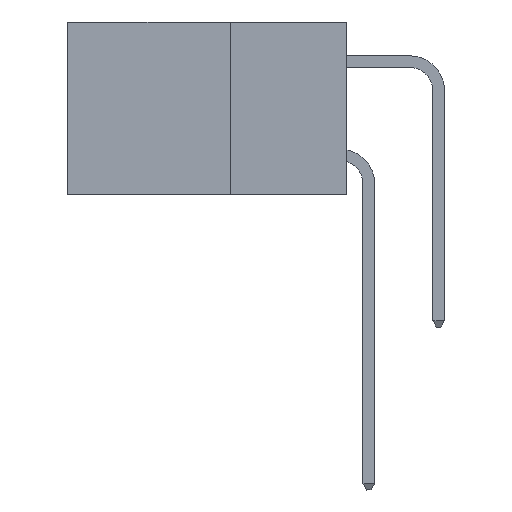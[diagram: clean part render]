
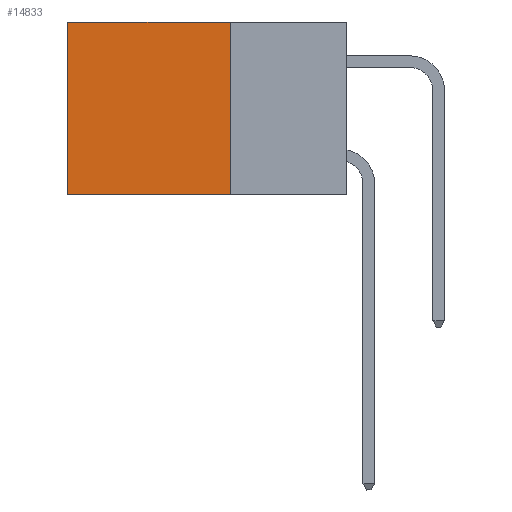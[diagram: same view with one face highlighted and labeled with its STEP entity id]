
A CAD part, left-side view. The second image highlights one B-rep face of the part: STEP entity #14833.
In plain terms, the highlighted planar face has unit normal (-1, 0, 0).
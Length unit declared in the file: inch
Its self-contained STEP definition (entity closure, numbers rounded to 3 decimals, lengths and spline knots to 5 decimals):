
#340 = ORIENTED_EDGE ( 'NONE', *, *, #6532, .T. ) ;
#3375 = VECTOR ( 'NONE', #14461, 39.37008 ) ;
#3875 = CARTESIAN_POINT ( 'NONE',  ( 0.2875, 0.6, 0. ) ) ;
#4419 = CARTESIAN_POINT ( 'NONE',  ( 0.2875, 0.6, 0. ) ) ;
#4865 = DIRECTION ( 'NONE',  ( 0., 0., -1. ) ) ;
#5165 = VECTOR ( 'NONE', #16690, 39.37008 ) ;
#5827 = VERTEX_POINT ( 'NONE', #13152 ) ;
#6100 = ORIENTED_EDGE ( 'NONE', *, *, #20010, .T. ) ;
#6532 = EDGE_CURVE ( 'NONE', #19696, #5827, #17785, .T. ) ;
#6641 = PLANE ( 'NONE',  #19958 ) ;
#7010 = LINE ( 'NONE', #12130, #10732 ) ;
#7231 = CARTESIAN_POINT ( 'NONE',  ( 0.2875, 0.25, 0. ) ) ;
#7678 = CARTESIAN_POINT ( 'NONE',  ( 0.2875, 0.25, 0. ) ) ;
#7954 = DIRECTION ( 'NONE',  ( 1., 0., 0. ) ) ;
#8232 = VERTEX_POINT ( 'NONE', #8935 ) ;
#8935 = CARTESIAN_POINT ( 'NONE',  ( 0.2875, 0.25, -0.37 ) ) ;
#8967 = DIRECTION ( 'NONE',  ( 0., 0., -1. ) ) ;
#9059 = CARTESIAN_POINT ( 'NONE',  ( 0.2875, 0.25, 0. ) ) ;
#9114 = DIRECTION ( 'NONE',  ( 0., 1., 0. ) ) ;
#9285 = LINE ( 'NONE', #17273, #3375 ) ;
#10732 = VECTOR ( 'NONE', #9114, 39.37008 ) ;
#10973 = VECTOR ( 'NONE', #8967, 39.37008 ) ;
#11355 = FACE_OUTER_BOUND ( 'NONE', #17914, .T. ) ;
#12130 = CARTESIAN_POINT ( 'NONE',  ( 0.2875, 0.25, -0.37 ) ) ;
#13152 = CARTESIAN_POINT ( 'NONE',  ( 0.2875, 0.6, -0.37 ) ) ;
#13173 = ORIENTED_EDGE ( 'NONE', *, *, #16865, .F. ) ;
#13844 = VERTEX_POINT ( 'NONE', #9059 ) ;
#14461 = DIRECTION ( 'NONE',  ( 0., 0., -1. ) ) ;
#14504 = LINE ( 'NONE', #7231, #5165 ) ;
#14833 = ADVANCED_FACE ( 'NONE', ( #11355 ), #6641, .F. ) ;
#15969 = ORIENTED_EDGE ( 'NONE', *, *, #16161, .F. ) ;
#16161 = EDGE_CURVE ( 'NONE', #13844, #8232, #9285, .T. ) ;
#16690 = DIRECTION ( 'NONE',  ( 0., 1., 0. ) ) ;
#16865 = EDGE_CURVE ( 'NONE', #8232, #5827, #7010, .T. ) ;
#17273 = CARTESIAN_POINT ( 'NONE',  ( 0.2875, 0.25, 0. ) ) ;
#17785 = LINE ( 'NONE', #4419, #10973 ) ;
#17914 = EDGE_LOOP ( 'NONE', ( #340, #13173, #15969, #6100 ) ) ;
#19696 = VERTEX_POINT ( 'NONE', #3875 ) ;
#19958 = AXIS2_PLACEMENT_3D ( 'NONE', #7678, #7954, #4865 ) ;
#20010 = EDGE_CURVE ( 'NONE', #13844, #19696, #14504, .T. ) ;
